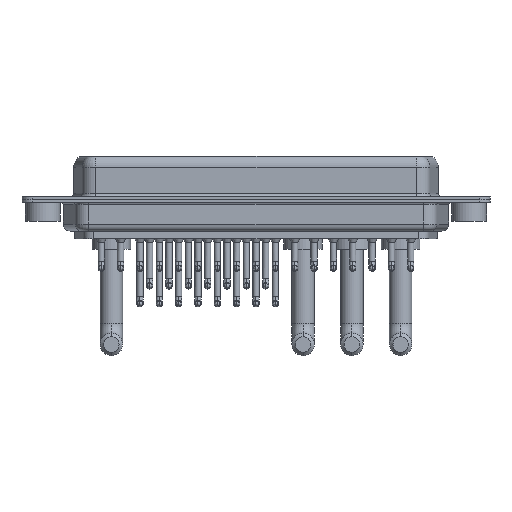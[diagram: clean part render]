
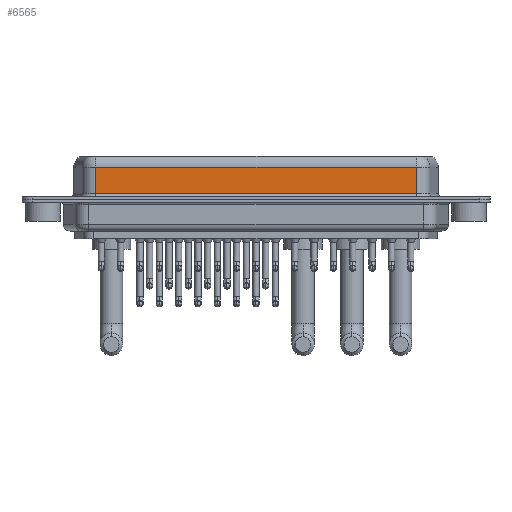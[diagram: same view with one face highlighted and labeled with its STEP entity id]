
A CAD part, front view. The second image highlights one B-rep face of the part: STEP entity #6565.
In plain terms, the highlighted planar face has unit normal (0, -1, 0).
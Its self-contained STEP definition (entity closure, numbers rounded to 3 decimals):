
#816 = ORIENTED_EDGE ( 'NONE', *, *, #13065, .T. ) ;
#984 = CARTESIAN_POINT ( 'NONE',  ( 7.59, -5.375, 0.9 ) ) ;
#1042 = DIRECTION ( 'NONE',  ( 0., 1., 0. ) ) ;
#1715 = CARTESIAN_POINT ( 'NONE',  ( 7.59, -5.375, 4.65 ) ) ;
#1726 = DIRECTION ( 'NONE',  ( -1., 0., 0. ) ) ;
#2710 = CARTESIAN_POINT ( 'NONE',  ( 53.41, -5.375, 0.9 ) ) ;
#2745 = EDGE_CURVE ( 'NONE', #6176, #21484, #22894, .T. ) ;
#3146 = VECTOR ( 'NONE', #1726, 1000. ) ;
#4170 = EDGE_CURVE ( 'NONE', #9864, #6176, #11808, .T. ) ;
#4400 = EDGE_LOOP ( 'NONE', ( #10117, #816, #11781, #11707 ) ) ;
#6176 = VERTEX_POINT ( 'NONE', #984 ) ;
#6565 = ADVANCED_FACE ( 'NONE', ( #18982 ), #14556, .F. ) ;
#6617 = VECTOR ( 'NONE', #13822, 1000. ) ;
#7596 = LINE ( 'NONE', #14273, #6617 ) ;
#8687 = CARTESIAN_POINT ( 'NONE',  ( 53.41, -5.375, 4.65 ) ) ;
#9191 = CARTESIAN_POINT ( 'NONE',  ( 53.41, -5.375, 4.65 ) ) ;
#9864 = VERTEX_POINT ( 'NONE', #1715 ) ;
#10117 = ORIENTED_EDGE ( 'NONE', *, *, #17015, .F. ) ;
#10123 = VECTOR ( 'NONE', #25443, 1000. ) ;
#10546 = CARTESIAN_POINT ( 'NONE',  ( 53.41, -5.375, 6.4 ) ) ;
#11707 = ORIENTED_EDGE ( 'NONE', *, *, #2745, .T. ) ;
#11781 = ORIENTED_EDGE ( 'NONE', *, *, #4170, .T. ) ;
#11808 = LINE ( 'NONE', #20837, #10123 ) ;
#13065 = EDGE_CURVE ( 'NONE', #22629, #9864, #28859, .T. ) ;
#13822 = DIRECTION ( 'NONE',  ( 0., 0., -1. ) ) ;
#14273 = CARTESIAN_POINT ( 'NONE',  ( 53.41, -5.375, 6.4 ) ) ;
#14556 = PLANE ( 'NONE',  #26553 ) ;
#17015 = EDGE_CURVE ( 'NONE', #22629, #21484, #7596, .T. ) ;
#18982 = FACE_OUTER_BOUND ( 'NONE', #4400, .T. ) ;
#20755 = VECTOR ( 'NONE', #27339, 1000. ) ;
#20837 = CARTESIAN_POINT ( 'NONE',  ( 7.59, -5.375, 6.4 ) ) ;
#21063 = CARTESIAN_POINT ( 'NONE',  ( 53.41, -5.375, 0.9 ) ) ;
#21209 = DIRECTION ( 'NONE',  ( 0., 0., 1. ) ) ;
#21484 = VERTEX_POINT ( 'NONE', #21063 ) ;
#22629 = VERTEX_POINT ( 'NONE', #9191 ) ;
#22894 = LINE ( 'NONE', #2710, #20755 ) ;
#25443 = DIRECTION ( 'NONE',  ( 0., 0., -1. ) ) ;
#26553 = AXIS2_PLACEMENT_3D ( 'NONE', #10546, #1042, #21209 ) ;
#27339 = DIRECTION ( 'NONE',  ( 1., 0., 0. ) ) ;
#28859 = LINE ( 'NONE', #8687, #3146 ) ;
